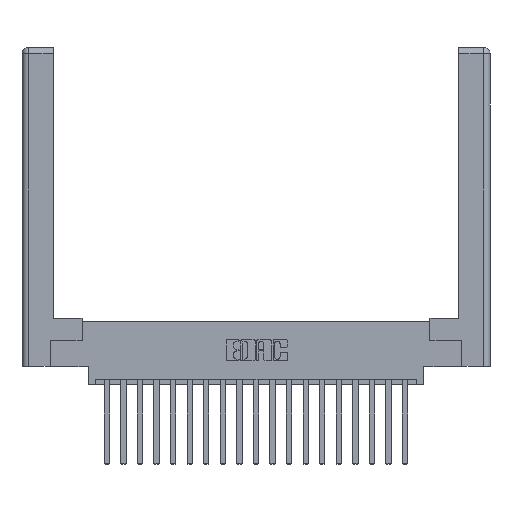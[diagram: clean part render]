
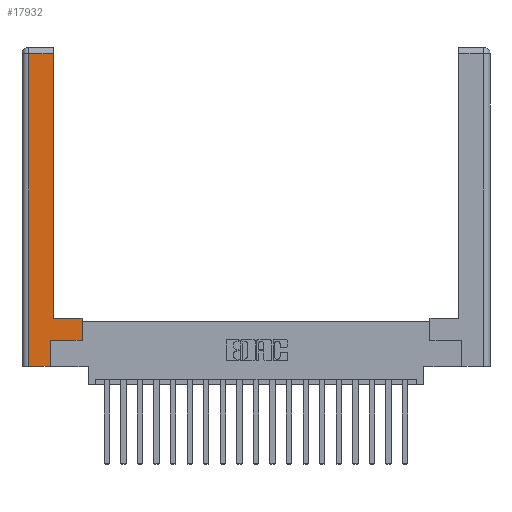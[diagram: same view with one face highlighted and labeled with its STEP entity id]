
A CAD part, top view. The second image highlights one B-rep face of the part: STEP entity #17932.
In plain terms, the highlighted planar face has unit normal (0, 0, 1).
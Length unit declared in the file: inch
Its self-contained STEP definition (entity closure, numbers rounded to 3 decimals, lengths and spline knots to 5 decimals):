
#618 = DIRECTION ( 'NONE',  ( 0., -1., 0. ) ) ;
#723 = VERTEX_POINT ( 'NONE', #13808 ) ;
#768 = EDGE_CURVE ( 'NONE', #12177, #3580, #9044, .T. ) ;
#1205 = ORIENTED_EDGE ( 'NONE', *, *, #768, .T. ) ;
#1860 = VECTOR ( 'NONE', #8680, 39.37008 ) ;
#2045 = LINE ( 'NONE', #8093, #6132 ) ;
#2433 = AXIS2_PLACEMENT_3D ( 'NONE', #8738, #13465, #11832 ) ;
#2759 = ORIENTED_EDGE ( 'NONE', *, *, #8713, .T. ) ;
#3492 = LINE ( 'NONE', #10145, #17956 ) ;
#3580 = VERTEX_POINT ( 'NONE', #6205 ) ;
#3587 = VECTOR ( 'NONE', #5556, 39.37008 ) ;
#3914 = VECTOR ( 'NONE', #17460, 39.37008 ) ;
#4027 = CARTESIAN_POINT ( 'NONE',  ( 0.265, 0., 0. ) ) ;
#4471 = VECTOR ( 'NONE', #18069, 39.37008 ) ;
#4511 = LINE ( 'NONE', #12383, #16538 ) ;
#4738 = CARTESIAN_POINT ( 'NONE',  ( 0.0615, 2.94, 0. ) ) ;
#5224 = CARTESIAN_POINT ( 'NONE',  ( 0.265, 0., 0. ) ) ;
#5556 = DIRECTION ( 'NONE',  ( -1., 0., 0. ) ) ;
#5773 = EDGE_CURVE ( 'NONE', #6608, #8383, #3492, .T. ) ;
#6132 = VECTOR ( 'NONE', #6980, 39.37008 ) ;
#6205 = CARTESIAN_POINT ( 'NONE',  ( 0.565, 0.245, 0. ) ) ;
#6235 = EDGE_LOOP ( 'NONE', ( #2759, #17503, #11903, #14679, #18988, #1205, #12901, #17468 ) ) ;
#6506 = EDGE_CURVE ( 'NONE', #15585, #12177, #2045, .T. ) ;
#6608 = VERTEX_POINT ( 'NONE', #17105 ) ;
#6871 = CARTESIAN_POINT ( 'NONE',  ( 0.0615, 2.94, 0. ) ) ;
#6919 = DIRECTION ( 'NONE',  ( -1., 0., 0. ) ) ;
#6980 = DIRECTION ( 'NONE',  ( 0., 1., 0. ) ) ;
#7777 = EDGE_CURVE ( 'NONE', #16643, #723, #15681, .T. ) ;
#7989 = CARTESIAN_POINT ( 'NONE',  ( 0.565, 0.245, 0. ) ) ;
#8093 = CARTESIAN_POINT ( 'NONE',  ( 0.265, 0.245, 0. ) ) ;
#8383 = VERTEX_POINT ( 'NONE', #16382 ) ;
#8680 = DIRECTION ( 'NONE',  ( 1., 0., 0. ) ) ;
#8713 = EDGE_CURVE ( 'NONE', #8383, #15161, #15015, .T. ) ;
#8738 = CARTESIAN_POINT ( 'NONE',  ( 0., 0., 0. ) ) ;
#8808 = FACE_OUTER_BOUND ( 'NONE', #6235, .T. ) ;
#9044 = LINE ( 'NONE', #7989, #3914 ) ;
#9958 = CARTESIAN_POINT ( 'NONE',  ( 0.0615, 0., 0. ) ) ;
#10145 = CARTESIAN_POINT ( 'NONE',  ( 0.295, 0.45, 0. ) ) ;
#11758 = PLANE ( 'NONE',  #2433 ) ;
#11832 = DIRECTION ( 'NONE',  ( -1., 0., 0. ) ) ;
#11903 = ORIENTED_EDGE ( 'NONE', *, *, #7777, .T. ) ;
#12177 = VERTEX_POINT ( 'NONE', #17383 ) ;
#12383 = CARTESIAN_POINT ( 'NONE',  ( 0.565, 0.45, 0. ) ) ;
#12901 = ORIENTED_EDGE ( 'NONE', *, *, #13846, .T. ) ;
#12946 = EDGE_CURVE ( 'NONE', #15161, #16643, #19530, .T. ) ;
#13465 = DIRECTION ( 'NONE',  ( 0., 0., -1. ) ) ;
#13808 = CARTESIAN_POINT ( 'NONE',  ( 0.0615, 0., 0. ) ) ;
#13846 = EDGE_CURVE ( 'NONE', #3580, #6608, #4511, .T. ) ;
#13914 = VECTOR ( 'NONE', #618, 39.37008 ) ;
#14086 = LINE ( 'NONE', #4027, #1860 ) ;
#14151 = EDGE_CURVE ( 'NONE', #723, #15585, #14086, .T. ) ;
#14173 = DIRECTION ( 'NONE',  ( 0., 1., 0. ) ) ;
#14679 = ORIENTED_EDGE ( 'NONE', *, *, #14151, .T. ) ;
#15015 = LINE ( 'NONE', #18005, #4471 ) ;
#15161 = VERTEX_POINT ( 'NONE', #19622 ) ;
#15585 = VERTEX_POINT ( 'NONE', #5224 ) ;
#15681 = LINE ( 'NONE', #9958, #13914 ) ;
#16382 = CARTESIAN_POINT ( 'NONE',  ( 0.295, 0.45, 0. ) ) ;
#16538 = VECTOR ( 'NONE', #14173, 39.37008 ) ;
#16643 = VERTEX_POINT ( 'NONE', #4738 ) ;
#17105 = CARTESIAN_POINT ( 'NONE',  ( 0.565, 0.45, 0. ) ) ;
#17383 = CARTESIAN_POINT ( 'NONE',  ( 0.265, 0.245, 0. ) ) ;
#17460 = DIRECTION ( 'NONE',  ( 1., 0., 0. ) ) ;
#17468 = ORIENTED_EDGE ( 'NONE', *, *, #5773, .T. ) ;
#17503 = ORIENTED_EDGE ( 'NONE', *, *, #12946, .T. ) ;
#17932 = ADVANCED_FACE ( 'NONE', ( #8808 ), #11758, .F. ) ;
#17956 = VECTOR ( 'NONE', #6919, 39.37008 ) ;
#18005 = CARTESIAN_POINT ( 'NONE',  ( 0.295, 3., 0. ) ) ;
#18069 = DIRECTION ( 'NONE',  ( 0., 1., 0. ) ) ;
#18988 = ORIENTED_EDGE ( 'NONE', *, *, #6506, .T. ) ;
#19530 = LINE ( 'NONE', #6871, #3587 ) ;
#19622 = CARTESIAN_POINT ( 'NONE',  ( 0.295, 2.94, 0. ) ) ;
